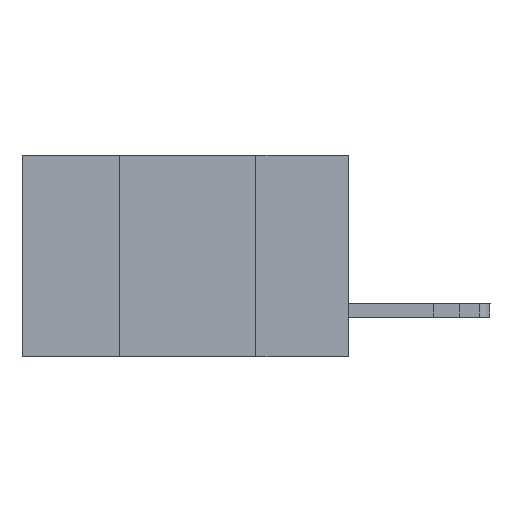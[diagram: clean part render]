
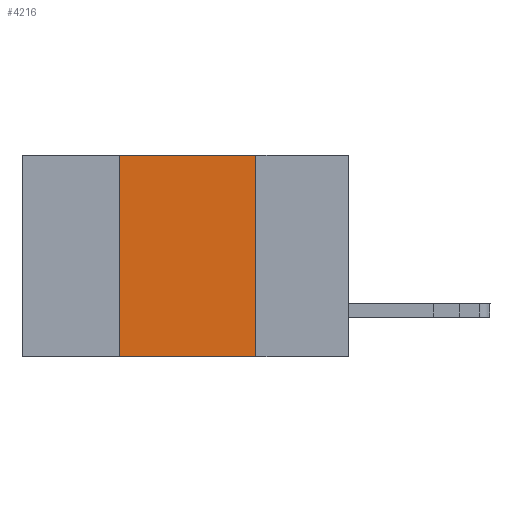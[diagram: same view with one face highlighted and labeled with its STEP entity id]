
A CAD part, left-side view. The second image highlights one B-rep face of the part: STEP entity #4216.
In plain terms, the highlighted planar face has unit normal (-1, 0, 0).
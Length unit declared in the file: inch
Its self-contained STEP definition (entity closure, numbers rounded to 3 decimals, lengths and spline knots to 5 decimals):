
#1017 = AXIS2_PLACEMENT_3D ( 'NONE', #9447, #9106, #9079 ) ;
#2482 = EDGE_CURVE ( 'NONE', #4455, #6808, #5210, .T. ) ;
#2510 = DIRECTION ( 'NONE',  ( 0., -1., 0. ) ) ;
#3281 = EDGE_LOOP ( 'NONE', ( #11255, #12025, #11348, #11013 ) ) ;
#3314 = EDGE_CURVE ( 'NONE', #4317, #6808, #5021, .T. ) ;
#3988 = VECTOR ( 'NONE', #5808, 39.37008 ) ;
#4157 = CARTESIAN_POINT ( 'NONE',  ( 0., 0.42, -0.37 ) ) ;
#4216 = ADVANCED_FACE ( 'NONE', ( #4616 ), #9193, .F. ) ;
#4317 = VERTEX_POINT ( 'NONE', #7872 ) ;
#4455 = VERTEX_POINT ( 'NONE', #6107 ) ;
#4616 = FACE_OUTER_BOUND ( 'NONE', #3281, .T. ) ;
#4855 = CARTESIAN_POINT ( 'NONE',  ( 0., 0.6, 0. ) ) ;
#5021 = LINE ( 'NONE', #5488, #10464 ) ;
#5210 = LINE ( 'NONE', #9360, #10983 ) ;
#5488 = CARTESIAN_POINT ( 'NONE',  ( 0., 0.17, -0.37 ) ) ;
#5648 = CARTESIAN_POINT ( 'NONE',  ( 0., 0.17, -0.37 ) ) ;
#5711 = EDGE_CURVE ( 'NONE', #4455, #6077, #10168, .T. ) ;
#5808 = DIRECTION ( 'NONE',  ( 0., 0., 1. ) ) ;
#6077 = VERTEX_POINT ( 'NONE', #8098 ) ;
#6107 = CARTESIAN_POINT ( 'NONE',  ( 0., 0.42, -0.37 ) ) ;
#6282 = EDGE_CURVE ( 'NONE', #6077, #4317, #14161, .T. ) ;
#6392 = DIRECTION ( 'NONE',  ( 0., 0., -1. ) ) ;
#6808 = VERTEX_POINT ( 'NONE', #5648 ) ;
#7872 = CARTESIAN_POINT ( 'NONE',  ( 0., 0.17, 0. ) ) ;
#8098 = CARTESIAN_POINT ( 'NONE',  ( 0., 0.42, 0. ) ) ;
#9079 = DIRECTION ( 'NONE',  ( 0., 0., -1. ) ) ;
#9106 = DIRECTION ( 'NONE',  ( 1., 0., 0. ) ) ;
#9108 = DIRECTION ( 'NONE',  ( 0., -1., 0. ) ) ;
#9193 = PLANE ( 'NONE',  #1017 ) ;
#9360 = CARTESIAN_POINT ( 'NONE',  ( 0., 0.6, -0.37 ) ) ;
#9447 = CARTESIAN_POINT ( 'NONE',  ( 0., 0.6, 0. ) ) ;
#10168 = LINE ( 'NONE', #4157, #3988 ) ;
#10464 = VECTOR ( 'NONE', #6392, 39.37008 ) ;
#10983 = VECTOR ( 'NONE', #9108, 39.37008 ) ;
#11013 = ORIENTED_EDGE ( 'NONE', *, *, #2482, .T. ) ;
#11255 = ORIENTED_EDGE ( 'NONE', *, *, #3314, .F. ) ;
#11348 = ORIENTED_EDGE ( 'NONE', *, *, #5711, .F. ) ;
#11376 = VECTOR ( 'NONE', #2510, 39.37008 ) ;
#12025 = ORIENTED_EDGE ( 'NONE', *, *, #6282, .F. ) ;
#14161 = LINE ( 'NONE', #4855, #11376 ) ;
